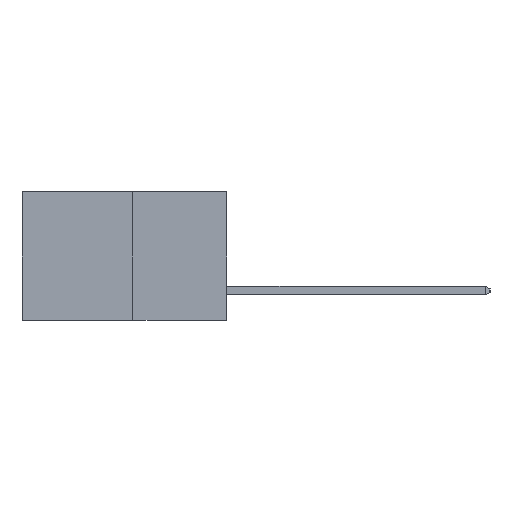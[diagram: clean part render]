
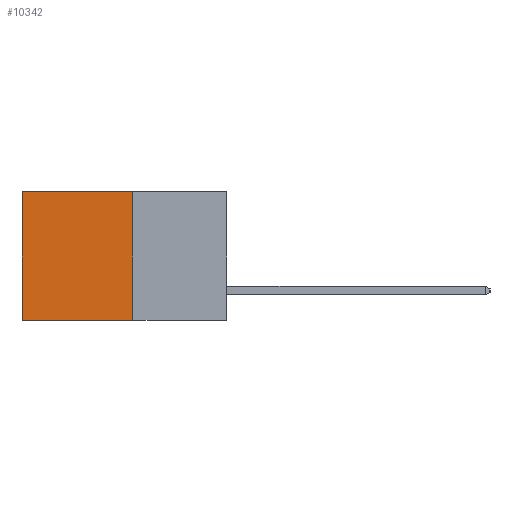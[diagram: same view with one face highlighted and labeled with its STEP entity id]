
A CAD part, left-side view. The second image highlights one B-rep face of the part: STEP entity #10342.
In plain terms, the highlighted planar face has unit normal (-1, 0, 0).
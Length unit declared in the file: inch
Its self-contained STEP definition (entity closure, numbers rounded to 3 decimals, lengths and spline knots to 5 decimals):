
#658 = ORIENTED_EDGE ( 'NONE', *, *, #7750, .F. ) ;
#1374 = VERTEX_POINT ( 'NONE', #5625 ) ;
#1634 = DIRECTION ( 'NONE',  ( 1., 0., 0. ) ) ;
#1671 = VECTOR ( 'NONE', #3578, 39.37008 ) ;
#1963 = VERTEX_POINT ( 'NONE', #9931 ) ;
#2743 = DIRECTION ( 'NONE',  ( 0., 0., -1. ) ) ;
#3240 = DIRECTION ( 'NONE',  ( 0., 1., 0. ) ) ;
#3578 = DIRECTION ( 'NONE',  ( 0., 0., -1. ) ) ;
#3593 = VECTOR ( 'NONE', #4934, 39.37008 ) ;
#3772 = EDGE_CURVE ( 'NONE', #11744, #1374, #8749, .T. ) ;
#4084 = CARTESIAN_POINT ( 'NONE',  ( 0.277, 0.27, -0.37 ) ) ;
#4398 = AXIS2_PLACEMENT_3D ( 'NONE', #9562, #1634, #10848 ) ;
#4410 = CARTESIAN_POINT ( 'NONE',  ( 0.277, 0.59, -0.37 ) ) ;
#4748 = VECTOR ( 'NONE', #3240, 39.37008 ) ;
#4934 = DIRECTION ( 'NONE',  ( 0., 1., 0. ) ) ;
#5487 = ORIENTED_EDGE ( 'NONE', *, *, #3772, .T. ) ;
#5625 = CARTESIAN_POINT ( 'NONE',  ( 0.277, 0.59, -0.37 ) ) ;
#5636 = CARTESIAN_POINT ( 'NONE',  ( 0.277, 0.59, 0. ) ) ;
#6856 = ORIENTED_EDGE ( 'NONE', *, *, #11431, .F. ) ;
#6902 = LINE ( 'NONE', #4084, #13483 ) ;
#7750 = EDGE_CURVE ( 'NONE', #10767, #1374, #10155, .T. ) ;
#7845 = EDGE_LOOP ( 'NONE', ( #5487, #658, #6856, #13779 ) ) ;
#8749 = LINE ( 'NONE', #4410, #1671 ) ;
#9106 = CARTESIAN_POINT ( 'NONE',  ( 0.277, 0.27, -0.37 ) ) ;
#9562 = CARTESIAN_POINT ( 'NONE',  ( 0.277, 0.27, -0.37 ) ) ;
#9931 = CARTESIAN_POINT ( 'NONE',  ( 0.277, 0.27, 0. ) ) ;
#10155 = LINE ( 'NONE', #11374, #3593 ) ;
#10342 = ADVANCED_FACE ( 'NONE', ( #13862 ), #15473, .F. ) ;
#10767 = VERTEX_POINT ( 'NONE', #9106 ) ;
#10848 = DIRECTION ( 'NONE',  ( 0., 0., -1. ) ) ;
#11374 = CARTESIAN_POINT ( 'NONE',  ( 0.277, 0.27, -0.37 ) ) ;
#11431 = EDGE_CURVE ( 'NONE', #1963, #10767, #6902, .T. ) ;
#11744 = VERTEX_POINT ( 'NONE', #5636 ) ;
#12023 = CARTESIAN_POINT ( 'NONE',  ( 0.277, 0.27, 0. ) ) ;
#13483 = VECTOR ( 'NONE', #2743, 39.37008 ) ;
#13779 = ORIENTED_EDGE ( 'NONE', *, *, #15956, .T. ) ;
#13862 = FACE_OUTER_BOUND ( 'NONE', #7845, .T. ) ;
#14714 = LINE ( 'NONE', #12023, #4748 ) ;
#15473 = PLANE ( 'NONE',  #4398 ) ;
#15956 = EDGE_CURVE ( 'NONE', #1963, #11744, #14714, .T. ) ;
